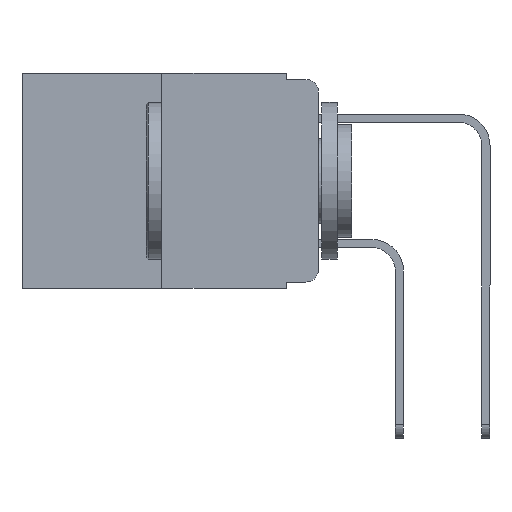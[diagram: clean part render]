
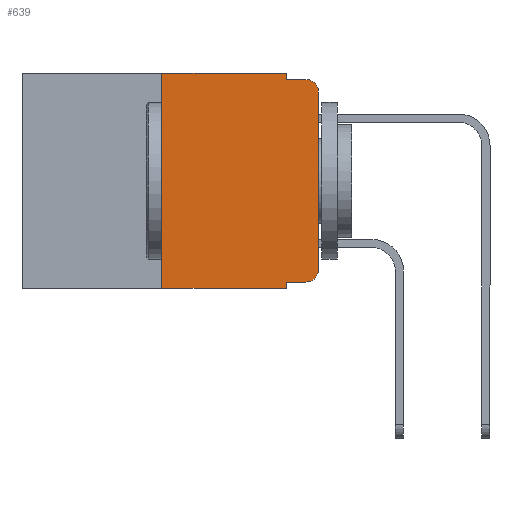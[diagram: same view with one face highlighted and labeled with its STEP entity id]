
A CAD part, left-side view. The second image highlights one B-rep face of the part: STEP entity #639.
In plain terms, the highlighted planar face has unit normal (-1, 0, 0).
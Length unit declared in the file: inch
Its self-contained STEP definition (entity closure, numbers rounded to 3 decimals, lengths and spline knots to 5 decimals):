
#639 = ADVANCED_FACE ( 'NONE', ( #6637 ), #4942, .F. ) ;
#680 = VERTEX_POINT ( 'NONE', #9691 ) ;
#785 = VECTOR ( 'NONE', #10202, 39.37008 ) ;
#1053 = LINE ( 'NONE', #3257, #10413 ) ;
#1090 = DIRECTION ( 'NONE',  ( 0., 0., -1. ) ) ;
#1248 = VERTEX_POINT ( 'NONE', #1666 ) ;
#1350 = VERTEX_POINT ( 'NONE', #10799 ) ;
#1437 = VERTEX_POINT ( 'NONE', #11877 ) ;
#1559 = EDGE_CURVE ( 'NONE', #1437, #4608, #4051, .T. ) ;
#1573 = ORIENTED_EDGE ( 'NONE', *, *, #10649, .T. ) ;
#1638 = CARTESIAN_POINT ( 'NONE',  ( 0., 0.02, -0.03 ) ) ;
#1653 = EDGE_CURVE ( 'NONE', #1248, #2683, #1053, .T. ) ;
#1666 = CARTESIAN_POINT ( 'NONE',  ( 0., 0.25, -0.343 ) ) ;
#1803 = CARTESIAN_POINT ( 'NONE',  ( 0., 0.051, -0.343 ) ) ;
#1860 = CARTESIAN_POINT ( 'NONE',  ( 0., 0.051, 0. ) ) ;
#1917 = ORIENTED_EDGE ( 'NONE', *, *, #11116, .F. ) ;
#2131 = DIRECTION ( 'NONE',  ( 0., -1., 0. ) ) ;
#2269 = ORIENTED_EDGE ( 'NONE', *, *, #1559, .T. ) ;
#2292 = VECTOR ( 'NONE', #11423, 39.37008 ) ;
#2496 = EDGE_CURVE ( 'NONE', #1248, #3648, #4522, .T. ) ;
#2683 = VERTEX_POINT ( 'NONE', #1803 ) ;
#2728 = DIRECTION ( 'NONE',  ( 0., 0., -1. ) ) ;
#2840 = VERTEX_POINT ( 'NONE', #8336 ) ;
#3257 = CARTESIAN_POINT ( 'NONE',  ( 0., 0.473, -0.343 ) ) ;
#3258 = VECTOR ( 'NONE', #5251, 39.37008 ) ;
#3402 = CARTESIAN_POINT ( 'NONE',  ( 0., 0.051, 0. ) ) ;
#3441 = CIRCLE ( 'NONE', #9019, 0.02 ) ;
#3550 = CARTESIAN_POINT ( 'NONE',  ( 0., 0.473, 0. ) ) ;
#3648 = VERTEX_POINT ( 'NONE', #4931 ) ;
#3732 = VECTOR ( 'NONE', #2131, 39.37008 ) ;
#3765 = DIRECTION ( 'NONE',  ( -1., 0., 0. ) ) ;
#3812 = DIRECTION ( 'NONE',  ( 0., -1., 0. ) ) ;
#4051 = LINE ( 'NONE', #9459, #3732 ) ;
#4425 = ORIENTED_EDGE ( 'NONE', *, *, #10664, .F. ) ;
#4522 = LINE ( 'NONE', #4576, #11158 ) ;
#4576 = CARTESIAN_POINT ( 'NONE',  ( 0., 0.25, 0. ) ) ;
#4608 = VERTEX_POINT ( 'NONE', #7875 ) ;
#4737 = ORIENTED_EDGE ( 'NONE', *, *, #2496, .F. ) ;
#4931 = CARTESIAN_POINT ( 'NONE',  ( 0., 0.25, 0. ) ) ;
#4942 = PLANE ( 'NONE',  #10193 ) ;
#5042 = ORIENTED_EDGE ( 'NONE', *, *, #10646, .T. ) ;
#5049 = LINE ( 'NONE', #1860, #7719 ) ;
#5060 = LINE ( 'NONE', #7256, #2292 ) ;
#5251 = DIRECTION ( 'NONE',  ( 0., -1., 0. ) ) ;
#6216 = VERTEX_POINT ( 'NONE', #8385 ) ;
#6634 = ORIENTED_EDGE ( 'NONE', *, *, #10357, .T. ) ;
#6637 = FACE_OUTER_BOUND ( 'NONE', #10632, .T. ) ;
#7193 = ORIENTED_EDGE ( 'NONE', *, *, #1653, .T. ) ;
#7256 = CARTESIAN_POINT ( 'NONE',  ( 0., 0., 0. ) ) ;
#7659 = DIRECTION ( 'NONE',  ( 1., 0., 0. ) ) ;
#7699 = VERTEX_POINT ( 'NONE', #3402 ) ;
#7719 = VECTOR ( 'NONE', #7739, 39.37008 ) ;
#7739 = DIRECTION ( 'NONE',  ( 0., 0., -1. ) ) ;
#7875 = CARTESIAN_POINT ( 'NONE',  ( 0., 0.02, -0.333 ) ) ;
#7911 = AXIS2_PLACEMENT_3D ( 'NONE', #9168, #3765, #10023 ) ;
#8127 = VECTOR ( 'NONE', #3812, 39.37008 ) ;
#8336 = CARTESIAN_POINT ( 'NONE',  ( 0., 0., -0.03 ) ) ;
#8385 = CARTESIAN_POINT ( 'NONE',  ( 0., 0.051, -0.01 ) ) ;
#8388 = CIRCLE ( 'NONE', #7911, 0.02 ) ;
#8389 = DIRECTION ( 'NONE',  ( -1., 0., 0. ) ) ;
#8502 = EDGE_CURVE ( 'NONE', #1437, #2683, #11242, .T. ) ;
#8506 = LINE ( 'NONE', #11245, #3258 ) ;
#8614 = CARTESIAN_POINT ( 'NONE',  ( 0., 0.051, 0. ) ) ;
#9019 = AXIS2_PLACEMENT_3D ( 'NONE', #1638, #8389, #2728 ) ;
#9168 = CARTESIAN_POINT ( 'NONE',  ( 0., 0.02, -0.313 ) ) ;
#9398 = ORIENTED_EDGE ( 'NONE', *, *, #8502, .F. ) ;
#9459 = CARTESIAN_POINT ( 'NONE',  ( 0., 0.051, -0.333 ) ) ;
#9691 = CARTESIAN_POINT ( 'NONE',  ( 0., 0., -0.313 ) ) ;
#9939 = DIRECTION ( 'NONE',  ( 0., -1., 0. ) ) ;
#10023 = DIRECTION ( 'NONE',  ( 0., 0., -1. ) ) ;
#10193 = AXIS2_PLACEMENT_3D ( 'NONE', #3550, #7659, #1090 ) ;
#10202 = DIRECTION ( 'NONE',  ( 0., 0., -1. ) ) ;
#10324 = LINE ( 'NONE', #11654, #8127 ) ;
#10357 = EDGE_CURVE ( 'NONE', #680, #2840, #5060, .T. ) ;
#10413 = VECTOR ( 'NONE', #9939, 39.37008 ) ;
#10632 = EDGE_LOOP ( 'NONE', ( #6634, #1573, #4425, #11347, #1917, #4737, #7193, #9398, #2269, #5042 ) ) ;
#10646 = EDGE_CURVE ( 'NONE', #4608, #680, #8388, .T. ) ;
#10649 = EDGE_CURVE ( 'NONE', #2840, #1350, #3441, .T. ) ;
#10664 = EDGE_CURVE ( 'NONE', #6216, #1350, #10324, .T. ) ;
#10799 = CARTESIAN_POINT ( 'NONE',  ( 0., 0.02, -0.01 ) ) ;
#11116 = EDGE_CURVE ( 'NONE', #3648, #7699, #8506, .T. ) ;
#11158 = VECTOR ( 'NONE', #11608, 39.37008 ) ;
#11242 = LINE ( 'NONE', #8614, #785 ) ;
#11245 = CARTESIAN_POINT ( 'NONE',  ( 0., 0.473, 0. ) ) ;
#11347 = ORIENTED_EDGE ( 'NONE', *, *, #11376, .F. ) ;
#11376 = EDGE_CURVE ( 'NONE', #7699, #6216, #5049, .T. ) ;
#11423 = DIRECTION ( 'NONE',  ( 0., 0., 1. ) ) ;
#11608 = DIRECTION ( 'NONE',  ( 0., 0., 1. ) ) ;
#11654 = CARTESIAN_POINT ( 'NONE',  ( 0., 0.051, -0.01 ) ) ;
#11877 = CARTESIAN_POINT ( 'NONE',  ( 0., 0.051, -0.333 ) ) ;
